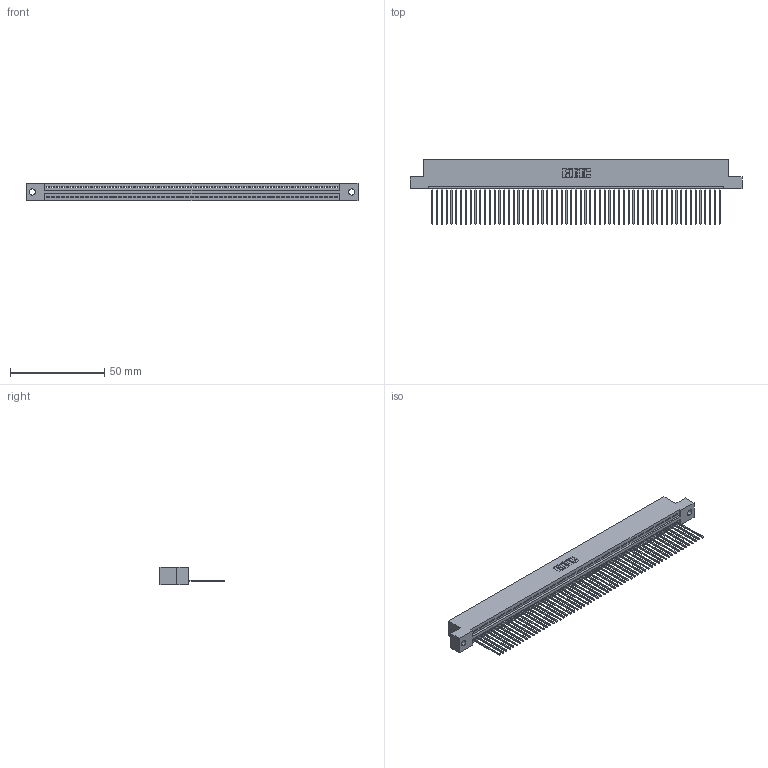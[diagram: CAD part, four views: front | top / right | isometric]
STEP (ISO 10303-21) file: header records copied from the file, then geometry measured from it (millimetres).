
FILE_DESCRIPTION (( 'STEP AP203' ), '1' );
FILE_NAME ('395-061-541-102.STEP', '2019-10-24T15:16:13', ( '' ), ( '' ), 'SwSTEP 2.0', 'SolidWorks 2016', '' );
FILE_SCHEMA (( 'CONFIG_CONTROL_DESIGN' ));
Length unit declared in the file: inch
Products named in the file (3): 345-292-001_345-293-141; 395-061-541-102; 345 Part_Flush Mounting Lugs - 0.128 Dia
Assembly tree (62 placements, depth 2):
  395-061-541-102
    345 Part_Flush Mounting Lugs - 0.128 Dia
    345-292-001_345-293-141  x61
Bounding box: 176.15 x 33.96 x 9.4 mm (x, y, z)
Volume: 17051.1 mm3; surface area: 23830.4 mm2
Topology: 62 solids, 62 shells, 3664 faces, 11077 edges, 7302 vertices
Faces by surface type: plane 2520, cylinder 1144
Entity records: 43373 total; most frequent: CARTESIAN_POINT 7519, ORIENTED_EDGE 7514, DIRECTION 6539, EDGE_CURVE 3757, VECTOR 3381, LINE 3381, VERTEX_POINT 2502, AXIS2_PLACEMENT_3D 1579
